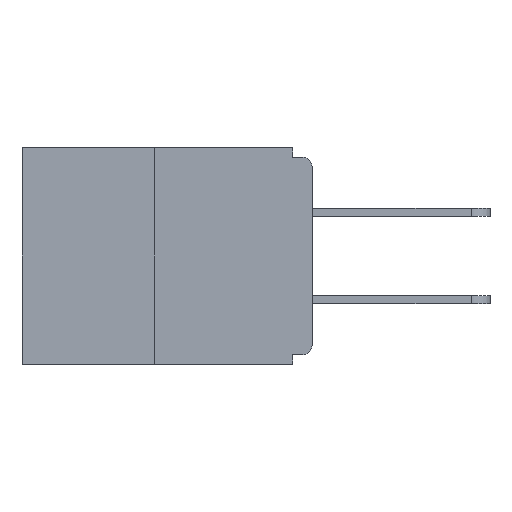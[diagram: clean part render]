
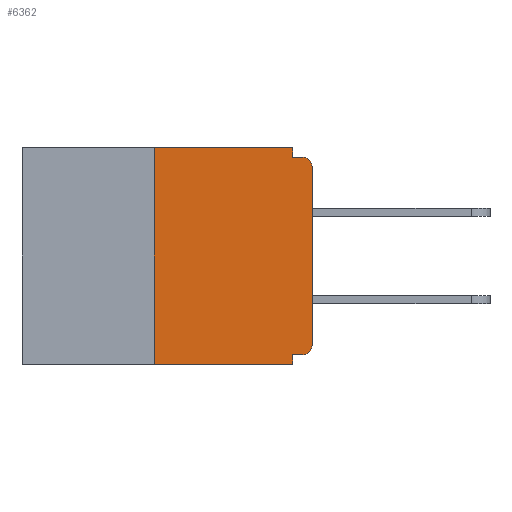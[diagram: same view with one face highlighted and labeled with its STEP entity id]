
A CAD part, left-side view. The second image highlights one B-rep face of the part: STEP entity #6362.
In plain terms, the highlighted planar face has unit normal (-1, 0, 0).
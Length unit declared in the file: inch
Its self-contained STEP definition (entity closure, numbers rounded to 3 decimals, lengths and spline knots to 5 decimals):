
#69 = VERTEX_POINT ( 'NONE', #5505 ) ;
#243 = EDGE_CURVE ( 'NONE', #6135, #13186, #12904, .T. ) ;
#612 = ORIENTED_EDGE ( 'NONE', *, *, #9862, .F. ) ;
#743 = VECTOR ( 'NONE', #1777, 39.37008 ) ;
#1101 = VECTOR ( 'NONE', #14101, 39.37008 ) ;
#1137 = FACE_OUTER_BOUND ( 'NONE', #6240, .T. ) ;
#1377 = CIRCLE ( 'NONE', #11869, 0.015 ) ;
#1526 = EDGE_CURVE ( 'NONE', #5552, #11543, #12458, .T. ) ;
#1700 = VECTOR ( 'NONE', #12190, 39.37008 ) ;
#1765 = CARTESIAN_POINT ( 'NONE',  ( 0., 0.031, -0.328 ) ) ;
#1777 = DIRECTION ( 'NONE',  ( 0., -1., 0. ) ) ;
#2118 = CARTESIAN_POINT ( 'NONE',  ( 0., 0.031, 0. ) ) ;
#3082 = CARTESIAN_POINT ( 'NONE',  ( 0., 0.031, 0. ) ) ;
#3164 = CARTESIAN_POINT ( 'NONE',  ( 0., 0.46, 0. ) ) ;
#3267 = ORIENTED_EDGE ( 'NONE', *, *, #1526, .F. ) ;
#3534 = CARTESIAN_POINT ( 'NONE',  ( 0., 0.25, 0. ) ) ;
#3604 = CARTESIAN_POINT ( 'NONE',  ( 0., 0.46, -0.343 ) ) ;
#3982 = CARTESIAN_POINT ( 'NONE',  ( 0., 0.46, 0. ) ) ;
#3992 = CARTESIAN_POINT ( 'NONE',  ( 0., 0.25, 0. ) ) ;
#4020 = LINE ( 'NONE', #15715, #11025 ) ;
#4061 = DIRECTION ( 'NONE',  ( 0., 0., 1. ) ) ;
#4197 = DIRECTION ( 'NONE',  ( 0., 0., -1. ) ) ;
#4329 = DIRECTION ( 'NONE',  ( -1., 0., 0. ) ) ;
#4561 = ORIENTED_EDGE ( 'NONE', *, *, #11458, .F. ) ;
#4756 = EDGE_CURVE ( 'NONE', #11543, #10756, #13808, .T. ) ;
#5105 = VECTOR ( 'NONE', #13446, 39.37008 ) ;
#5287 = CARTESIAN_POINT ( 'NONE',  ( 0., 0.015, -0.03 ) ) ;
#5341 = LINE ( 'NONE', #3604, #1101 ) ;
#5418 = ORIENTED_EDGE ( 'NONE', *, *, #11623, .F. ) ;
#5505 = CARTESIAN_POINT ( 'NONE',  ( 0., 0.015, -0.015 ) ) ;
#5552 = VERTEX_POINT ( 'NONE', #6124 ) ;
#5556 = ORIENTED_EDGE ( 'NONE', *, *, #243, .T. ) ;
#5706 = CARTESIAN_POINT ( 'NONE',  ( 0., 0.015, -0.313 ) ) ;
#5934 = LINE ( 'NONE', #3082, #5105 ) ;
#6124 = CARTESIAN_POINT ( 'NONE',  ( 0., 0.25, -0.343 ) ) ;
#6135 = VERTEX_POINT ( 'NONE', #15964 ) ;
#6240 = EDGE_LOOP ( 'NONE', ( #14302, #3267, #15303, #4561, #5418, #5556, #6507, #9528, #14366, #612 ) ) ;
#6362 = ADVANCED_FACE ( 'NONE', ( #1137 ), #15872, .F. ) ;
#6507 = ORIENTED_EDGE ( 'NONE', *, *, #14866, .T. ) ;
#6992 = EDGE_CURVE ( 'NONE', #5552, #16646, #5341, .T. ) ;
#7059 = CARTESIAN_POINT ( 'NONE',  ( 0., 0., -0.313 ) ) ;
#7072 = CARTESIAN_POINT ( 'NONE',  ( 0., 0., -0.015 ) ) ;
#7157 = LINE ( 'NONE', #7072, #1700 ) ;
#7614 = EDGE_CURVE ( 'NONE', #9893, #69, #7157, .T. ) ;
#7981 = DIRECTION ( 'NONE',  ( 1., 0., 0. ) ) ;
#8089 = DIRECTION ( 'NONE',  ( -1., 0., 0. ) ) ;
#8144 = VECTOR ( 'NONE', #4061, 39.37008 ) ;
#8316 = AXIS2_PLACEMENT_3D ( 'NONE', #5706, #4329, #15701 ) ;
#8566 = VECTOR ( 'NONE', #16559, 39.37008 ) ;
#9100 = CARTESIAN_POINT ( 'NONE',  ( 0., 0., -0.03 ) ) ;
#9487 = CARTESIAN_POINT ( 'NONE',  ( 0., 0.031, -0.343 ) ) ;
#9497 = CARTESIAN_POINT ( 'NONE',  ( 0., 0., -0.328 ) ) ;
#9528 = ORIENTED_EDGE ( 'NONE', *, *, #16898, .T. ) ;
#9819 = VERTEX_POINT ( 'NONE', #1765 ) ;
#9862 = EDGE_CURVE ( 'NONE', #10756, #9893, #5934, .T. ) ;
#9893 = VERTEX_POINT ( 'NONE', #14913 ) ;
#9947 = AXIS2_PLACEMENT_3D ( 'NONE', #3982, #7981, #13214 ) ;
#10756 = VERTEX_POINT ( 'NONE', #2118 ) ;
#11025 = VECTOR ( 'NONE', #14532, 39.37008 ) ;
#11224 = VECTOR ( 'NONE', #16055, 39.37008 ) ;
#11451 = LINE ( 'NONE', #15625, #8144 ) ;
#11458 = EDGE_CURVE ( 'NONE', #9819, #16646, #4020, .T. ) ;
#11543 = VERTEX_POINT ( 'NONE', #3992 ) ;
#11623 = EDGE_CURVE ( 'NONE', #6135, #9819, #14484, .T. ) ;
#11869 = AXIS2_PLACEMENT_3D ( 'NONE', #5287, #8089, #4197 ) ;
#12190 = DIRECTION ( 'NONE',  ( 0., -1., 0. ) ) ;
#12458 = LINE ( 'NONE', #3534, #8566 ) ;
#12904 = CIRCLE ( 'NONE', #8316, 0.015 ) ;
#13186 = VERTEX_POINT ( 'NONE', #7059 ) ;
#13214 = DIRECTION ( 'NONE',  ( 0., 0., -1. ) ) ;
#13446 = DIRECTION ( 'NONE',  ( 0., 0., -1. ) ) ;
#13808 = LINE ( 'NONE', #3164, #743 ) ;
#14101 = DIRECTION ( 'NONE',  ( 0., -1., 0. ) ) ;
#14302 = ORIENTED_EDGE ( 'NONE', *, *, #4756, .F. ) ;
#14366 = ORIENTED_EDGE ( 'NONE', *, *, #7614, .F. ) ;
#14484 = LINE ( 'NONE', #9497, #11224 ) ;
#14532 = DIRECTION ( 'NONE',  ( 0., 0., -1. ) ) ;
#14866 = EDGE_CURVE ( 'NONE', #13186, #15516, #11451, .T. ) ;
#14913 = CARTESIAN_POINT ( 'NONE',  ( 0., 0.031, -0.015 ) ) ;
#15303 = ORIENTED_EDGE ( 'NONE', *, *, #6992, .T. ) ;
#15516 = VERTEX_POINT ( 'NONE', #9100 ) ;
#15625 = CARTESIAN_POINT ( 'NONE',  ( 0., 0., 0. ) ) ;
#15701 = DIRECTION ( 'NONE',  ( 0., 0., -1. ) ) ;
#15715 = CARTESIAN_POINT ( 'NONE',  ( 0., 0.031, -0.343 ) ) ;
#15872 = PLANE ( 'NONE',  #9947 ) ;
#15964 = CARTESIAN_POINT ( 'NONE',  ( 0., 0.015, -0.328 ) ) ;
#16055 = DIRECTION ( 'NONE',  ( 0., 1., 0. ) ) ;
#16559 = DIRECTION ( 'NONE',  ( 0., 0., 1. ) ) ;
#16646 = VERTEX_POINT ( 'NONE', #9487 ) ;
#16898 = EDGE_CURVE ( 'NONE', #15516, #69, #1377, .T. ) ;
